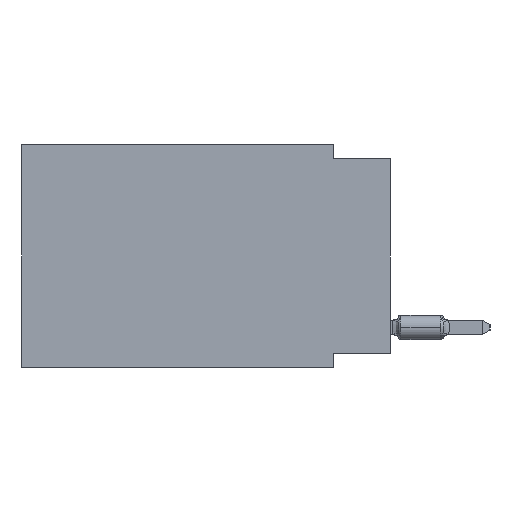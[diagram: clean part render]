
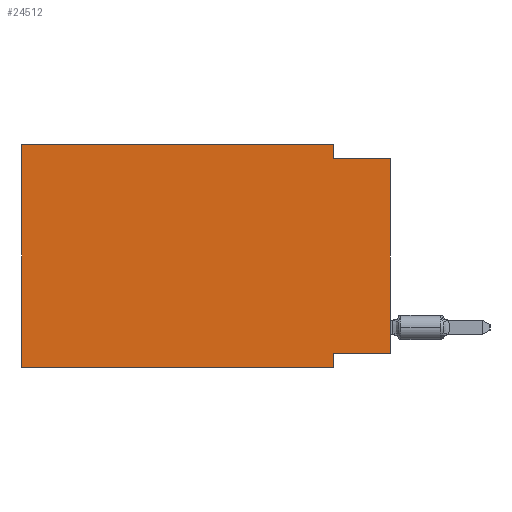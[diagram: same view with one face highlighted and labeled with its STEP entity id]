
A CAD part, left-side view. The second image highlights one B-rep face of the part: STEP entity #24512.
In plain terms, the highlighted planar face has unit normal (-1, 0, 0).
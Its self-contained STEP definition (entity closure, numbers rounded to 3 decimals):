
#228 = CARTESIAN_POINT ( 'NONE',  ( 0., 2.54, -0.635 ) ) ;
#365 = DIRECTION ( 'NONE',  ( 0., 0., 1. ) ) ;
#584 = LINE ( 'NONE', #27777, #78847 ) ;
#1306 = VERTEX_POINT ( 'NONE', #3235 ) ;
#1713 = ORIENTED_EDGE ( 'NONE', *, *, #25062, .T. ) ;
#3213 = DIRECTION ( 'NONE',  ( 0., -1., 0. ) ) ;
#3235 = CARTESIAN_POINT ( 'NONE',  ( 0., 2.54, -9.906 ) ) ;
#3684 = PLANE ( 'NONE',  #76791 ) ;
#4731 = VERTEX_POINT ( 'NONE', #67898 ) ;
#7127 = DIRECTION ( 'NONE',  ( 0., -1., 0. ) ) ;
#8998 = ORIENTED_EDGE ( 'NONE', *, *, #47039, .F. ) ;
#9019 = CARTESIAN_POINT ( 'NONE',  ( 0., 0., -9.271 ) ) ;
#9094 = ORIENTED_EDGE ( 'NONE', *, *, #81515, .T. ) ;
#9560 = EDGE_CURVE ( 'NONE', #4731, #21662, #584, .T. ) ;
#11385 = ORIENTED_EDGE ( 'NONE', *, *, #9560, .F. ) ;
#13808 = LINE ( 'NONE', #40969, #69594 ) ;
#16468 = CARTESIAN_POINT ( 'NONE',  ( 0., 2.54, -9.906 ) ) ;
#18894 = LINE ( 'NONE', #52304, #50161 ) ;
#20432 = CARTESIAN_POINT ( 'NONE',  ( 0., 16.383, 0. ) ) ;
#21662 = VERTEX_POINT ( 'NONE', #76347 ) ;
#24480 = LINE ( 'NONE', #16468, #49382 ) ;
#24512 = ADVANCED_FACE ( 'NONE', ( #31752 ), #3684, .F. ) ;
#25062 = EDGE_CURVE ( 'NONE', #59515, #1306, #26282, .T. ) ;
#26282 = LINE ( 'NONE', #86859, #54541 ) ;
#26374 = LINE ( 'NONE', #80729, #52421 ) ;
#27777 = CARTESIAN_POINT ( 'NONE',  ( 0., 16.383, 0. ) ) ;
#28494 = VERTEX_POINT ( 'NONE', #70727 ) ;
#30365 = DIRECTION ( 'NONE',  ( 0., 0., 1. ) ) ;
#31026 = VERTEX_POINT ( 'NONE', #228 ) ;
#31752 = FACE_OUTER_BOUND ( 'NONE', #66212, .T. ) ;
#40969 = CARTESIAN_POINT ( 'NONE',  ( 0., 0., -0.635 ) ) ;
#46442 = ORIENTED_EDGE ( 'NONE', *, *, #65674, .F. ) ;
#46753 = DIRECTION ( 'NONE',  ( 0., -1., 0. ) ) ;
#47039 = EDGE_CURVE ( 'NONE', #21662, #31026, #18894, .T. ) ;
#49382 = VECTOR ( 'NONE', #51634, 1000. ) ;
#50161 = VECTOR ( 'NONE', #86177, 1000. ) ;
#51634 = DIRECTION ( 'NONE',  ( 0., 0., -1. ) ) ;
#51784 = CARTESIAN_POINT ( 'NONE',  ( 0., 16.383, 0. ) ) ;
#52304 = CARTESIAN_POINT ( 'NONE',  ( 0., 2.54, 0. ) ) ;
#52421 = VECTOR ( 'NONE', #74485, 1000. ) ;
#54541 = VECTOR ( 'NONE', #46753, 1000. ) ;
#58042 = DIRECTION ( 'NONE',  ( 0., 0., -1. ) ) ;
#59515 = VERTEX_POINT ( 'NONE', #69739 ) ;
#60596 = VECTOR ( 'NONE', #365, 1000. ) ;
#61897 = CARTESIAN_POINT ( 'NONE',  ( 0., 2.54, -9.271 ) ) ;
#62228 = ORIENTED_EDGE ( 'NONE', *, *, #85462, .F. ) ;
#62343 = EDGE_CURVE ( 'NONE', #59515, #4731, #81489, .T. ) ;
#62737 = VECTOR ( 'NONE', #30365, 1000. ) ;
#65674 = EDGE_CURVE ( 'NONE', #84377, #1306, #24480, .T. ) ;
#66212 = EDGE_LOOP ( 'NONE', ( #9094, #62228, #8998, #11385, #82330, #1713, #46442, #69149 ) ) ;
#67898 = CARTESIAN_POINT ( 'NONE',  ( 0., 16.383, 0. ) ) ;
#69149 = ORIENTED_EDGE ( 'NONE', *, *, #78734, .F. ) ;
#69594 = VECTOR ( 'NONE', #7127, 1000. ) ;
#69739 = CARTESIAN_POINT ( 'NONE',  ( 0., 16.383, -9.906 ) ) ;
#70727 = CARTESIAN_POINT ( 'NONE',  ( 0., 0., -0.635 ) ) ;
#71354 = CARTESIAN_POINT ( 'NONE',  ( 0., 0., 0. ) ) ;
#71866 = DIRECTION ( 'NONE',  ( 1., 0., 0. ) ) ;
#74485 = DIRECTION ( 'NONE',  ( 0., 1., 0. ) ) ;
#76347 = CARTESIAN_POINT ( 'NONE',  ( 0., 2.54, 0. ) ) ;
#76791 = AXIS2_PLACEMENT_3D ( 'NONE', #51784, #71866, #58042 ) ;
#77610 = LINE ( 'NONE', #71354, #62737 ) ;
#78734 = EDGE_CURVE ( 'NONE', #83834, #84377, #26374, .T. ) ;
#78847 = VECTOR ( 'NONE', #3213, 1000. ) ;
#80729 = CARTESIAN_POINT ( 'NONE',  ( 0., 0., -9.271 ) ) ;
#81489 = LINE ( 'NONE', #20432, #60596 ) ;
#81515 = EDGE_CURVE ( 'NONE', #83834, #28494, #77610, .T. ) ;
#82330 = ORIENTED_EDGE ( 'NONE', *, *, #62343, .F. ) ;
#83834 = VERTEX_POINT ( 'NONE', #9019 ) ;
#84377 = VERTEX_POINT ( 'NONE', #61897 ) ;
#85462 = EDGE_CURVE ( 'NONE', #31026, #28494, #13808, .T. ) ;
#86177 = DIRECTION ( 'NONE',  ( 0., 0., -1. ) ) ;
#86859 = CARTESIAN_POINT ( 'NONE',  ( 0., 16.383, -9.906 ) ) ;
